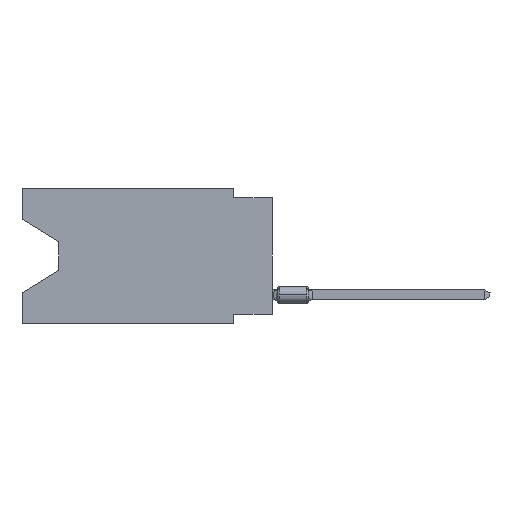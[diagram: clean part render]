
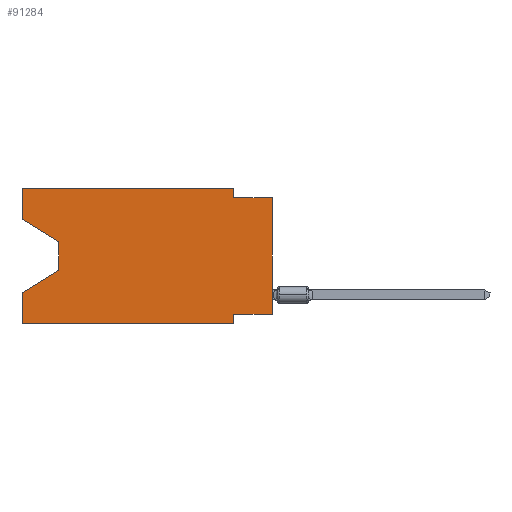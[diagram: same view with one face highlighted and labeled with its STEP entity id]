
A CAD part, left-side view. The second image highlights one B-rep face of the part: STEP entity #91284.
In plain terms, the highlighted planar face has unit normal (-1, 0, 0).
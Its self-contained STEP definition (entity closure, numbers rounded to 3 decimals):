
#9 = LINE ( 'NONE', #115885, #47763 ) ;
#19 = DIRECTION ( 'NONE',  ( 0., 1., 0. ) ) ;
#357 = CARTESIAN_POINT ( 'NONE',  ( 0., 13.97, -3.505 ) ) ;
#1452 = ORIENTED_EDGE ( 'NONE', *, *, #59040, .F. ) ;
#3710 = CARTESIAN_POINT ( 'NONE',  ( 0., 2.54, -8.89 ) ) ;
#4387 = PLANE ( 'NONE',  #89572 ) ;
#4469 = VERTEX_POINT ( 'NONE', #24447 ) ;
#6160 = EDGE_CURVE ( 'NONE', #39128, #47495, #87283, .T. ) ;
#6786 = ORIENTED_EDGE ( 'NONE', *, *, #82519, .F. ) ;
#8048 = CARTESIAN_POINT ( 'NONE',  ( 0., 16.383, -2.038 ) ) ;
#9106 = CARTESIAN_POINT ( 'NONE',  ( 0., 16.383, 0. ) ) ;
#9177 = DIRECTION ( 'NONE',  ( 0., 0., -1. ) ) ;
#9767 = LINE ( 'NONE', #357, #31385 ) ;
#15123 = VERTEX_POINT ( 'NONE', #92234 ) ;
#15387 = CARTESIAN_POINT ( 'NONE',  ( 0., 16.383, 0. ) ) ;
#16507 = LINE ( 'NONE', #61195, #79583 ) ;
#17066 = EDGE_CURVE ( 'NONE', #100459, #103573, #33225, .T. ) ;
#17482 = VECTOR ( 'NONE', #52105, 1000. ) ;
#19672 = LINE ( 'NONE', #9106, #91320 ) ;
#19913 = DIRECTION ( 'NONE',  ( 0., 0., 1. ) ) ;
#20671 = EDGE_CURVE ( 'NONE', #21087, #100459, #66494, .T. ) ;
#20970 = CARTESIAN_POINT ( 'NONE',  ( 0., 16.383, -6.852 ) ) ;
#21087 = VERTEX_POINT ( 'NONE', #21670 ) ;
#21456 = DIRECTION ( 'NONE',  ( 1., 0., 0. ) ) ;
#21670 = CARTESIAN_POINT ( 'NONE',  ( 0., 2.54, 0. ) ) ;
#24363 = CARTESIAN_POINT ( 'NONE',  ( 0., 16.383, -8.89 ) ) ;
#24447 = CARTESIAN_POINT ( 'NONE',  ( 0., 2.54, -8.255 ) ) ;
#24455 = LINE ( 'NONE', #77998, #17482 ) ;
#26013 = VERTEX_POINT ( 'NONE', #3710 ) ;
#26476 = DIRECTION ( 'NONE',  ( 0., 0., -1. ) ) ;
#27380 = CARTESIAN_POINT ( 'NONE',  ( 0., 0., -0.635 ) ) ;
#30276 = DIRECTION ( 'NONE',  ( 0., 0., -1. ) ) ;
#30353 = LINE ( 'NONE', #103262, #104097 ) ;
#31385 = VECTOR ( 'NONE', #9177, 1000. ) ;
#31495 = DIRECTION ( 'NONE',  ( 0., 0.855, -0.519 ) ) ;
#32006 = FACE_OUTER_BOUND ( 'NONE', #100580, .T. ) ;
#32134 = ORIENTED_EDGE ( 'NONE', *, *, #35433, .T. ) ;
#33225 = LINE ( 'NONE', #53212, #93785 ) ;
#33812 = CARTESIAN_POINT ( 'NONE',  ( 0., 2.54, -0.635 ) ) ;
#35433 = EDGE_CURVE ( 'NONE', #47495, #90794, #9767, .T. ) ;
#39128 = VERTEX_POINT ( 'NONE', #8048 ) ;
#39317 = VERTEX_POINT ( 'NONE', #98583 ) ;
#42383 = ORIENTED_EDGE ( 'NONE', *, *, #74313, .F. ) ;
#43566 = VERTEX_POINT ( 'NONE', #24363 ) ;
#44635 = CARTESIAN_POINT ( 'NONE',  ( 0., 16.383, 0. ) ) ;
#47495 = VERTEX_POINT ( 'NONE', #100328 ) ;
#47505 = CARTESIAN_POINT ( 'NONE',  ( 0., 13.97, -5.385 ) ) ;
#47763 = VECTOR ( 'NONE', #26476, 1000. ) ;
#48287 = DIRECTION ( 'NONE',  ( 0., 0., -1. ) ) ;
#51254 = DIRECTION ( 'NONE',  ( 0., 0., 1. ) ) ;
#52105 = DIRECTION ( 'NONE',  ( 0., -1., 0. ) ) ;
#53212 = CARTESIAN_POINT ( 'NONE',  ( 0., 0., -0.635 ) ) ;
#53453 = LINE ( 'NONE', #44635, #71074 ) ;
#54967 = DIRECTION ( 'NONE',  ( 0., -1., 0. ) ) ;
#55387 = VECTOR ( 'NONE', #106390, 1000. ) ;
#57697 = DIRECTION ( 'NONE',  ( 0., -0.855, -0.519 ) ) ;
#59040 = EDGE_CURVE ( 'NONE', #43566, #73144, #95932, .T. ) ;
#59436 = CARTESIAN_POINT ( 'NONE',  ( 0., 16.383, -2.038 ) ) ;
#60255 = VECTOR ( 'NONE', #48287, 1000. ) ;
#61195 = CARTESIAN_POINT ( 'NONE',  ( 0., 0., -8.255 ) ) ;
#62214 = ORIENTED_EDGE ( 'NONE', *, *, #84022, .T. ) ;
#65686 = VECTOR ( 'NONE', #57697, 1000. ) ;
#66494 = LINE ( 'NONE', #84726, #60255 ) ;
#69727 = ORIENTED_EDGE ( 'NONE', *, *, #86793, .F. ) ;
#71074 = VECTOR ( 'NONE', #19913, 1000. ) ;
#72018 = EDGE_CURVE ( 'NONE', #90794, #73144, #30353, .T. ) ;
#73144 = VERTEX_POINT ( 'NONE', #20970 ) ;
#74313 = EDGE_CURVE ( 'NONE', #4469, #26013, #9, .T. ) ;
#75025 = ORIENTED_EDGE ( 'NONE', *, *, #17066, .F. ) ;
#77998 = CARTESIAN_POINT ( 'NONE',  ( 0., 16.383, -8.89 ) ) ;
#79357 = CARTESIAN_POINT ( 'NONE',  ( 0., 0., 0. ) ) ;
#79388 = ORIENTED_EDGE ( 'NONE', *, *, #6160, .T. ) ;
#79583 = VECTOR ( 'NONE', #19, 1000. ) ;
#80506 = LINE ( 'NONE', #79357, #55387 ) ;
#82519 = EDGE_CURVE ( 'NONE', #39317, #4469, #16507, .T. ) ;
#83343 = ORIENTED_EDGE ( 'NONE', *, *, #112730, .T. ) ;
#84022 = EDGE_CURVE ( 'NONE', #39317, #103573, #80506, .T. ) ;
#84378 = CARTESIAN_POINT ( 'NONE',  ( 0., 16.383, 0. ) ) ;
#84726 = CARTESIAN_POINT ( 'NONE',  ( 0., 2.54, 0. ) ) ;
#86793 = EDGE_CURVE ( 'NONE', #15123, #21087, #19672, .T. ) ;
#87283 = LINE ( 'NONE', #59436, #65686 ) ;
#88542 = VECTOR ( 'NONE', #51254, 1000. ) ;
#89572 = AXIS2_PLACEMENT_3D ( 'NONE', #84378, #21456, #30276 ) ;
#90210 = ORIENTED_EDGE ( 'NONE', *, *, #93671, .F. ) ;
#90794 = VERTEX_POINT ( 'NONE', #47505 ) ;
#91284 = ADVANCED_FACE ( 'NONE', ( #32006 ), #4387, .F. ) ;
#91320 = VECTOR ( 'NONE', #54967, 1000. ) ;
#92234 = CARTESIAN_POINT ( 'NONE',  ( 0., 16.383, 0. ) ) ;
#93671 = EDGE_CURVE ( 'NONE', #39128, #15123, #53453, .T. ) ;
#93785 = VECTOR ( 'NONE', #96155, 1000. ) ;
#95932 = LINE ( 'NONE', #15387, #88542 ) ;
#96155 = DIRECTION ( 'NONE',  ( 0., -1., 0. ) ) ;
#98583 = CARTESIAN_POINT ( 'NONE',  ( 0., 0., -8.255 ) ) ;
#100328 = CARTESIAN_POINT ( 'NONE',  ( 0., 13.97, -3.505 ) ) ;
#100459 = VERTEX_POINT ( 'NONE', #33812 ) ;
#100580 = EDGE_LOOP ( 'NONE', ( #79388, #32134, #109947, #1452, #83343, #42383, #6786, #62214, #75025, #102133, #69727, #90210 ) ) ;
#102133 = ORIENTED_EDGE ( 'NONE', *, *, #20671, .F. ) ;
#103262 = CARTESIAN_POINT ( 'NONE',  ( 0., 13.97, -5.385 ) ) ;
#103573 = VERTEX_POINT ( 'NONE', #27380 ) ;
#104097 = VECTOR ( 'NONE', #31495, 1000. ) ;
#106390 = DIRECTION ( 'NONE',  ( 0., 0., 1. ) ) ;
#109947 = ORIENTED_EDGE ( 'NONE', *, *, #72018, .T. ) ;
#112730 = EDGE_CURVE ( 'NONE', #43566, #26013, #24455, .T. ) ;
#115885 = CARTESIAN_POINT ( 'NONE',  ( 0., 2.54, -8.89 ) ) ;
